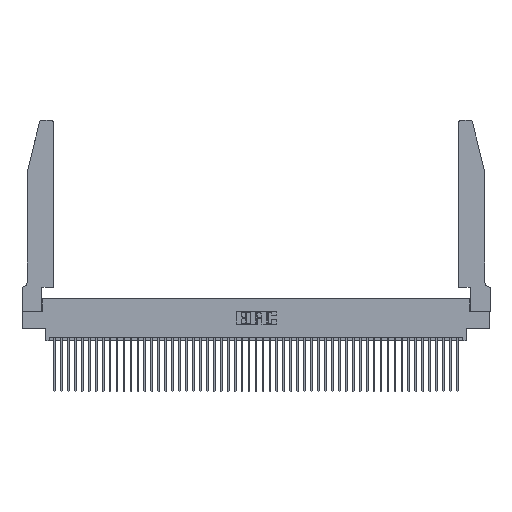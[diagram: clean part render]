
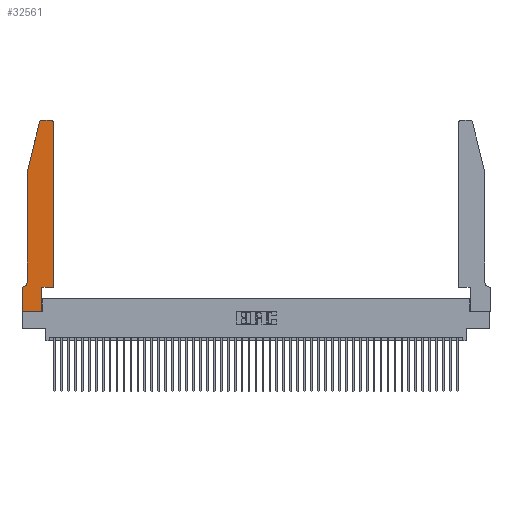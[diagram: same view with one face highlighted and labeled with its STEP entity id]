
A CAD part, top view. The second image highlights one B-rep face of the part: STEP entity #32561.
In plain terms, the highlighted planar face has unit normal (0, 0, 1).
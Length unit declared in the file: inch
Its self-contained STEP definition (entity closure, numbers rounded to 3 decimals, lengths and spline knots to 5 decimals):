
#36 = CARTESIAN_POINT ( 'NONE',  ( 0.4505, 0.35, 0.37 ) ) ;
#694 = VERTEX_POINT ( 'NONE', #24365 ) ;
#1434 = DIRECTION ( 'NONE',  ( 0., 0., 1. ) ) ;
#3514 = CARTESIAN_POINT ( 'NONE',  ( 0., 0., 0.37 ) ) ;
#3934 = LINE ( 'NONE', #7299, #32939 ) ;
#4104 = LINE ( 'NONE', #30437, #23251 ) ;
#4288 = EDGE_CURVE ( 'NONE', #22592, #46036, #20623, .T. ) ;
#5366 = CARTESIAN_POINT ( 'NONE',  ( 0., 0.35, 0.37 ) ) ;
#5405 = EDGE_LOOP ( 'NONE', ( #46871, #35135, #23513, #8546, #47394, #35095, #47963, #18700, #14496, #29802, #18031, #34879 ) ) ;
#5435 = VERTEX_POINT ( 'NONE', #17356 ) ;
#6334 = DIRECTION ( 'NONE',  ( 1., 0., 0. ) ) ;
#6618 = CIRCLE ( 'NONE', #45910, 0.03 ) ;
#7299 = CARTESIAN_POINT ( 'NONE',  ( 0.2865, 0.35, 0.37 ) ) ;
#7899 = EDGE_CURVE ( 'NONE', #694, #42145, #34525, .T. ) ;
#8546 = ORIENTED_EDGE ( 'NONE', *, *, #36256, .T. ) ;
#8964 = LINE ( 'NONE', #17766, #17979 ) ;
#9260 = EDGE_CURVE ( 'NONE', #19554, #40410, #6618, .T. ) ;
#9405 = FACE_OUTER_BOUND ( 'NONE', #5405, .T. ) ;
#9565 = VECTOR ( 'NONE', #29708, 39.37008 ) ;
#10701 = CARTESIAN_POINT ( 'NONE',  ( 0.4205, 2.72, 0.37 ) ) ;
#11106 = CARTESIAN_POINT ( 'NONE',  ( 0.284, 2.72, 0.37 ) ) ;
#13146 = VERTEX_POINT ( 'NONE', #28681 ) ;
#14496 = ORIENTED_EDGE ( 'NONE', *, *, #40186, .T. ) ;
#14604 = DIRECTION ( 'NONE',  ( 1., 0., 0. ) ) ;
#14989 = DIRECTION ( 'NONE',  ( 1., 0., 0. ) ) ;
#15216 = CARTESIAN_POINT ( 'NONE',  ( 0.0055, 0.42, 0.37 ) ) ;
#15218 = VECTOR ( 'NONE', #20703, 39.37008 ) ;
#16269 = EDGE_CURVE ( 'NONE', #42145, #19554, #19771, .T. ) ;
#16752 = PLANE ( 'NONE',  #30758 ) ;
#17042 = CARTESIAN_POINT ( 'NONE',  ( 0.0755, 0.42, 0.37 ) ) ;
#17094 = EDGE_CURVE ( 'NONE', #32876, #22592, #4104, .T. ) ;
#17356 = CARTESIAN_POINT ( 'NONE',  ( 0.2865, 0.35, 0.37 ) ) ;
#17766 = CARTESIAN_POINT ( 'NONE',  ( 0., 0., 0.37 ) ) ;
#17979 = VECTOR ( 'NONE', #6334, 39.37008 ) ;
#18031 = ORIENTED_EDGE ( 'NONE', *, *, #48640, .T. ) ;
#18700 = ORIENTED_EDGE ( 'NONE', *, *, #18774, .T. ) ;
#18774 = EDGE_CURVE ( 'NONE', #46036, #13146, #8964, .T. ) ;
#19051 = DIRECTION ( 'NONE',  ( -1., 0., 0. ) ) ;
#19128 = CARTESIAN_POINT ( 'NONE',  ( 0.0755, 2., 0.37 ) ) ;
#19554 = VERTEX_POINT ( 'NONE', #25588 ) ;
#19771 = LINE ( 'NONE', #25971, #9565 ) ;
#20623 = LINE ( 'NONE', #3514, #40446 ) ;
#20703 = DIRECTION ( 'NONE',  ( 1., 0., 0. ) ) ;
#21461 = CARTESIAN_POINT ( 'NONE',  ( 0.4505, 0.35, 0.37 ) ) ;
#21900 = LINE ( 'NONE', #35834, #40539 ) ;
#22592 = VERTEX_POINT ( 'NONE', #5366 ) ;
#22994 = DIRECTION ( 'NONE',  ( 0., 1., 0. ) ) ;
#23251 = VECTOR ( 'NONE', #34169, 39.37008 ) ;
#23255 = EDGE_CURVE ( 'NONE', #5435, #40635, #45101, .T. ) ;
#23513 = ORIENTED_EDGE ( 'NONE', *, *, #25904, .T. ) ;
#24356 = CARTESIAN_POINT ( 'NONE',  ( 0., 0.35, 0.37 ) ) ;
#24365 = CARTESIAN_POINT ( 'NONE',  ( 0.4505, 2.72, 0.37 ) ) ;
#25204 = CARTESIAN_POINT ( 'NONE',  ( 0.4205, 2.75, 0.37 ) ) ;
#25588 = CARTESIAN_POINT ( 'NONE',  ( 0.284, 2.75, 0.37 ) ) ;
#25904 = EDGE_CURVE ( 'NONE', #40410, #26956, #21900, .T. ) ;
#25971 = CARTESIAN_POINT ( 'NONE',  ( 0.2605, 2.75, 0.37 ) ) ;
#26956 = VERTEX_POINT ( 'NONE', #19128 ) ;
#28087 = DIRECTION ( 'NONE',  ( 1., 0., 0. ) ) ;
#28681 = CARTESIAN_POINT ( 'NONE',  ( 0.2865, 0., 0.37 ) ) ;
#29708 = DIRECTION ( 'NONE',  ( -1., 0., 0. ) ) ;
#29802 = ORIENTED_EDGE ( 'NONE', *, *, #23255, .T. ) ;
#30079 = DIRECTION ( 'NONE',  ( 0., -1., 0. ) ) ;
#30170 = DIRECTION ( 'NONE',  ( 0., 1., 0. ) ) ;
#30437 = CARTESIAN_POINT ( 'NONE',  ( 0.0755, 0.35, 0.37 ) ) ;
#30758 = AXIS2_PLACEMENT_3D ( 'NONE', #24356, #1434, #28087 ) ;
#30949 = EDGE_CURVE ( 'NONE', #48381, #32876, #34878, .T. ) ;
#31255 = DIRECTION ( 'NONE',  ( 0., -1., 0. ) ) ;
#32561 = ADVANCED_FACE ( 'NONE', ( #9405 ), #16752, .T. ) ;
#32876 = VERTEX_POINT ( 'NONE', #48450 ) ;
#32939 = VECTOR ( 'NONE', #30170, 39.37008 ) ;
#33545 = LINE ( 'NONE', #36, #42273 ) ;
#34169 = DIRECTION ( 'NONE',  ( -1., 0., 0. ) ) ;
#34525 = CIRCLE ( 'NONE', #43678, 0.03 ) ;
#34878 = CIRCLE ( 'NONE', #47911, 0.07 ) ;
#34879 = ORIENTED_EDGE ( 'NONE', *, *, #7899, .T. ) ;
#35010 = CARTESIAN_POINT ( 'NONE',  ( 0., 0., 0.37 ) ) ;
#35070 = LINE ( 'NONE', #42302, #42644 ) ;
#35095 = ORIENTED_EDGE ( 'NONE', *, *, #17094, .T. ) ;
#35135 = ORIENTED_EDGE ( 'NONE', *, *, #9260, .T. ) ;
#35834 = CARTESIAN_POINT ( 'NONE',  ( 0.0755, 2., 0.37 ) ) ;
#36256 = EDGE_CURVE ( 'NONE', #26956, #48381, #35070, .T. ) ;
#37023 = DIRECTION ( 'NONE',  ( 0., 0., 1. ) ) ;
#37397 = DIRECTION ( 'NONE',  ( 0., 0., 1. ) ) ;
#38738 = CARTESIAN_POINT ( 'NONE',  ( 0.25487, 2.72718, 0.37 ) ) ;
#39268 = CARTESIAN_POINT ( 'NONE',  ( 0.4505, 0.35, 0.37 ) ) ;
#39588 = DIRECTION ( 'NONE',  ( -0.239, -0.971, 0. ) ) ;
#40186 = EDGE_CURVE ( 'NONE', #13146, #5435, #3934, .T. ) ;
#40410 = VERTEX_POINT ( 'NONE', #38738 ) ;
#40446 = VECTOR ( 'NONE', #30079, 39.37008 ) ;
#40539 = VECTOR ( 'NONE', #39588, 39.37008 ) ;
#40635 = VERTEX_POINT ( 'NONE', #21461 ) ;
#41391 = DIRECTION ( 'NONE',  ( 0., 0., -1. ) ) ;
#42145 = VERTEX_POINT ( 'NONE', #25204 ) ;
#42273 = VECTOR ( 'NONE', #22994, 39.37008 ) ;
#42302 = CARTESIAN_POINT ( 'NONE',  ( 0.0755, 2., 0.37 ) ) ;
#42644 = VECTOR ( 'NONE', #31255, 39.37008 ) ;
#43678 = AXIS2_PLACEMENT_3D ( 'NONE', #10701, #37023, #14604 ) ;
#45101 = LINE ( 'NONE', #39268, #15218 ) ;
#45910 = AXIS2_PLACEMENT_3D ( 'NONE', #11106, #37397, #14989 ) ;
#46036 = VERTEX_POINT ( 'NONE', #35010 ) ;
#46871 = ORIENTED_EDGE ( 'NONE', *, *, #16269, .T. ) ;
#47394 = ORIENTED_EDGE ( 'NONE', *, *, #30949, .T. ) ;
#47911 = AXIS2_PLACEMENT_3D ( 'NONE', #15216, #41391, #19051 ) ;
#47963 = ORIENTED_EDGE ( 'NONE', *, *, #4288, .T. ) ;
#48381 = VERTEX_POINT ( 'NONE', #17042 ) ;
#48450 = CARTESIAN_POINT ( 'NONE',  ( 0.0055, 0.35, 0.37 ) ) ;
#48640 = EDGE_CURVE ( 'NONE', #40635, #694, #33545, .T. ) ;
